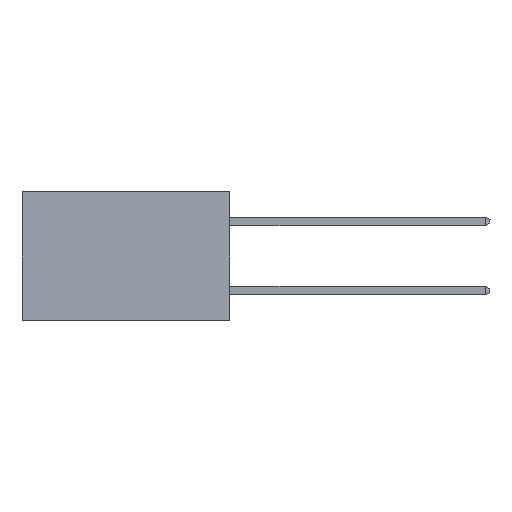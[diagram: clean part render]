
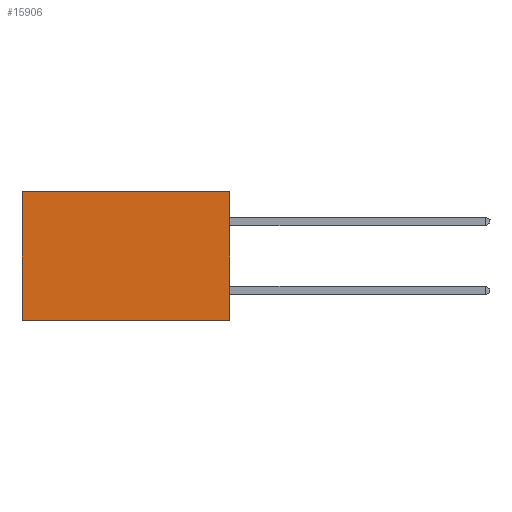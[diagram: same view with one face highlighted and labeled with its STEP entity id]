
A CAD part, left-side view. The second image highlights one B-rep face of the part: STEP entity #15906.
In plain terms, the highlighted planar face has unit normal (-1, 0, 0).
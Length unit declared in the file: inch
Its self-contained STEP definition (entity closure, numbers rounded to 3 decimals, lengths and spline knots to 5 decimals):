
#843 = EDGE_CURVE ( 'NONE', #8694, #10335, #11962, .T. ) ;
#1120 = CARTESIAN_POINT ( 'NONE',  ( 0.2615, 0.6, -0.37 ) ) ;
#1678 = FACE_OUTER_BOUND ( 'NONE', #4058, .T. ) ;
#3633 = EDGE_CURVE ( 'NONE', #10335, #4852, #8228, .T. ) ;
#3698 = ORIENTED_EDGE ( 'NONE', *, *, #843, .T. ) ;
#4058 = EDGE_LOOP ( 'NONE', ( #15272, #18743, #17180, #3698 ) ) ;
#4376 = CARTESIAN_POINT ( 'NONE',  ( 0.2615, 0., -0.37 ) ) ;
#4852 = VERTEX_POINT ( 'NONE', #1120 ) ;
#5030 = AXIS2_PLACEMENT_3D ( 'NONE', #14288, #19764, #11591 ) ;
#5588 = CARTESIAN_POINT ( 'NONE',  ( 0.2615, 0., 0. ) ) ;
#6979 = LINE ( 'NONE', #13371, #18628 ) ;
#7314 = CARTESIAN_POINT ( 'NONE',  ( 0.2615, 0., 0. ) ) ;
#7987 = PLANE ( 'NONE',  #5030 ) ;
#8228 = LINE ( 'NONE', #13184, #16777 ) ;
#8241 = CARTESIAN_POINT ( 'NONE',  ( 0.2615, 0., -0.37 ) ) ;
#8694 = VERTEX_POINT ( 'NONE', #5588 ) ;
#9439 = EDGE_CURVE ( 'NONE', #8694, #14071, #9582, .T. ) ;
#9582 = LINE ( 'NONE', #8241, #18637 ) ;
#9767 = DIRECTION ( 'NONE',  ( 0., 0., -1. ) ) ;
#10335 = VERTEX_POINT ( 'NONE', #12549 ) ;
#10495 = VECTOR ( 'NONE', #19836, 39.37008 ) ;
#11591 = DIRECTION ( 'NONE',  ( 0., 0., -1. ) ) ;
#11962 = LINE ( 'NONE', #7314, #10495 ) ;
#12549 = CARTESIAN_POINT ( 'NONE',  ( 0.2615, 0.6, 0. ) ) ;
#13184 = CARTESIAN_POINT ( 'NONE',  ( 0.2615, 0.6, -0.37 ) ) ;
#13371 = CARTESIAN_POINT ( 'NONE',  ( 0.2615, 0., -0.37 ) ) ;
#14071 = VERTEX_POINT ( 'NONE', #4376 ) ;
#14140 = DIRECTION ( 'NONE',  ( 0., 0., -1. ) ) ;
#14288 = CARTESIAN_POINT ( 'NONE',  ( 0.2615, 0., -0.37 ) ) ;
#15272 = ORIENTED_EDGE ( 'NONE', *, *, #3633, .T. ) ;
#15906 = ADVANCED_FACE ( 'NONE', ( #1678 ), #7987, .F. ) ;
#16777 = VECTOR ( 'NONE', #9767, 39.37008 ) ;
#16798 = DIRECTION ( 'NONE',  ( 0., 1., 0. ) ) ;
#17180 = ORIENTED_EDGE ( 'NONE', *, *, #9439, .F. ) ;
#18628 = VECTOR ( 'NONE', #16798, 39.37008 ) ;
#18637 = VECTOR ( 'NONE', #14140, 39.37008 ) ;
#18743 = ORIENTED_EDGE ( 'NONE', *, *, #19296, .F. ) ;
#19296 = EDGE_CURVE ( 'NONE', #14071, #4852, #6979, .T. ) ;
#19764 = DIRECTION ( 'NONE',  ( 1., 0., 0. ) ) ;
#19836 = DIRECTION ( 'NONE',  ( 0., 1., 0. ) ) ;
